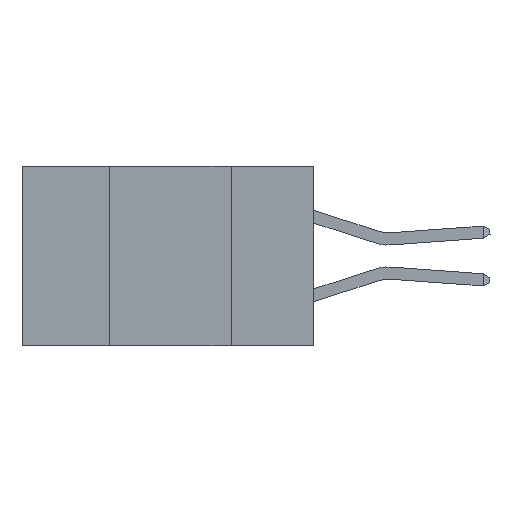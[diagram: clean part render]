
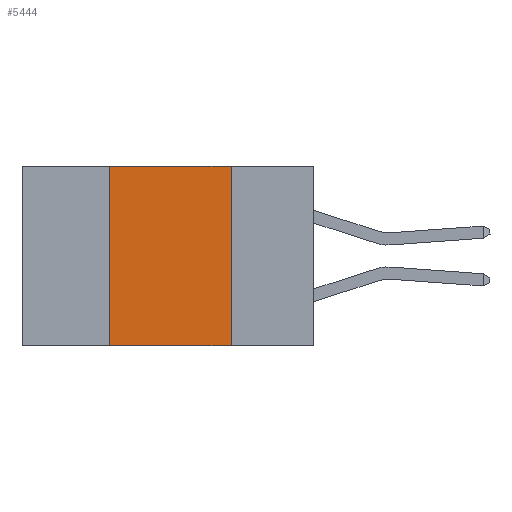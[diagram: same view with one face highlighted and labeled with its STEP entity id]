
A CAD part, left-side view. The second image highlights one B-rep face of the part: STEP entity #5444.
In plain terms, the highlighted planar face has unit normal (-1, 0, 0).
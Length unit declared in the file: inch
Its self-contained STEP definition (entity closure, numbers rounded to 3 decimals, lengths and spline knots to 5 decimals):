
#592 = ORIENTED_EDGE ( 'NONE', *, *, #16173, .F. ) ;
#1294 = VERTEX_POINT ( 'NONE', #2340 ) ;
#1904 = EDGE_CURVE ( 'NONE', #12511, #18650, #8839, .T. ) ;
#2340 = CARTESIAN_POINT ( 'NONE',  ( 0., 0.42, 0. ) ) ;
#2541 = DIRECTION ( 'NONE',  ( 0., 0., -1. ) ) ;
#3986 = DIRECTION ( 'NONE',  ( 1., 0., 0. ) ) ;
#4124 = DIRECTION ( 'NONE',  ( 0., 0., -1. ) ) ;
#4401 = EDGE_CURVE ( 'NONE', #1294, #12666, #15828, .T. ) ;
#5051 = LINE ( 'NONE', #11066, #15272 ) ;
#5336 = DIRECTION ( 'NONE',  ( 0., -1., 0. ) ) ;
#5444 = ADVANCED_FACE ( 'NONE', ( #14487 ), #14392, .F. ) ;
#6912 = CARTESIAN_POINT ( 'NONE',  ( 0., 0.17, 0. ) ) ;
#6962 = VECTOR ( 'NONE', #5336, 39.37008 ) ;
#8519 = VECTOR ( 'NONE', #12074, 39.37008 ) ;
#8839 = LINE ( 'NONE', #14908, #8519 ) ;
#9043 = CARTESIAN_POINT ( 'NONE',  ( 0., 0.17, -0.37 ) ) ;
#9672 = CARTESIAN_POINT ( 'NONE',  ( 0., 0.6, 0. ) ) ;
#9943 = VECTOR ( 'NONE', #4124, 39.37008 ) ;
#10373 = CARTESIAN_POINT ( 'NONE',  ( 0., 0.6, 0. ) ) ;
#11066 = CARTESIAN_POINT ( 'NONE',  ( 0., 0.42, 0. ) ) ;
#11261 = EDGE_CURVE ( 'NONE', #12666, #18650, #15892, .T. ) ;
#11503 = CARTESIAN_POINT ( 'NONE',  ( 0., 0.17, 0. ) ) ;
#12069 = ORIENTED_EDGE ( 'NONE', *, *, #1904, .T. ) ;
#12074 = DIRECTION ( 'NONE',  ( 0., -1., 0. ) ) ;
#12511 = VERTEX_POINT ( 'NONE', #18263 ) ;
#12666 = VERTEX_POINT ( 'NONE', #6912 ) ;
#14392 = PLANE ( 'NONE',  #17636 ) ;
#14487 = FACE_OUTER_BOUND ( 'NONE', #16401, .T. ) ;
#14908 = CARTESIAN_POINT ( 'NONE',  ( 0., 0.6, -0.37 ) ) ;
#15272 = VECTOR ( 'NONE', #17007, 39.37008 ) ;
#15828 = LINE ( 'NONE', #9672, #6962 ) ;
#15892 = LINE ( 'NONE', #11503, #9943 ) ;
#16173 = EDGE_CURVE ( 'NONE', #12511, #1294, #5051, .T. ) ;
#16401 = EDGE_LOOP ( 'NONE', ( #16470, #19295, #592, #12069 ) ) ;
#16470 = ORIENTED_EDGE ( 'NONE', *, *, #11261, .F. ) ;
#17007 = DIRECTION ( 'NONE',  ( 0., 0., 1. ) ) ;
#17636 = AXIS2_PLACEMENT_3D ( 'NONE', #10373, #3986, #2541 ) ;
#18263 = CARTESIAN_POINT ( 'NONE',  ( 0., 0.42, -0.37 ) ) ;
#18650 = VERTEX_POINT ( 'NONE', #9043 ) ;
#19295 = ORIENTED_EDGE ( 'NONE', *, *, #4401, .F. ) ;
